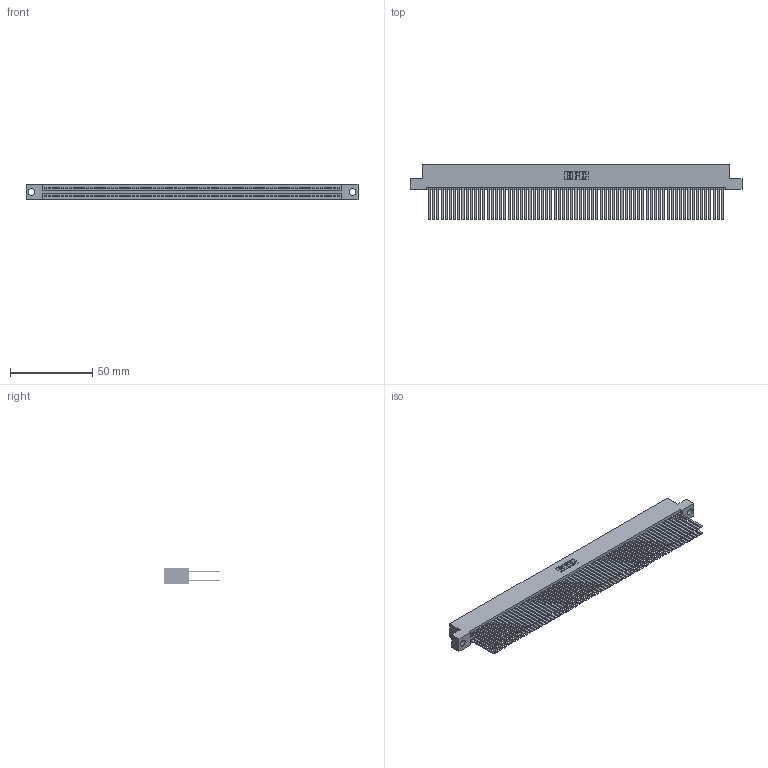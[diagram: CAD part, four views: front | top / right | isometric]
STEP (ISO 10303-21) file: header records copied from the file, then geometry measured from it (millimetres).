
FILE_DESCRIPTION (( 'STEP AP203' ), '1' );
FILE_NAME ('345-142-544-204.STEP', '2021-05-26T02:05:35', ( '' ), ( '' ), 'SwSTEP 2.0', 'SolidWorks 2020', '' );
FILE_SCHEMA (( 'CONFIG_CONTROL_DESIGN' ));
Length unit declared in the file: inch
Products named in the file (3): 345 Part_Flush Mounting Lugs - 0.156 Dia-TI; 345-292-001_345-293-144; 345-142-544-204
Assembly tree (143 placements, depth 2):
  345-142-544-204
    345 Part_Flush Mounting Lugs - 0.156 Dia-TI
    345-292-001_345-293-144  x142
Bounding box: 201.55 x 33.96 x 9.4 mm (x, y, z)
Volume: 21732.5 mm3; surface area: 38371.7 mm2
Topology: 143 solids, 143 shells, 6388 faces, 18979 edges, 12462 vertices
Faces by surface type: plane 4212, cylinder 2176
Entity records: 52039 total; most frequent: CARTESIAN_POINT 8698, ORIENTED_EDGE 8630, DIRECTION 7631, EDGE_CURVE 4315, LINE 3903, VECTOR 3903, VERTEX_POINT 2874, AXIS2_PLACEMENT_3D 1864
